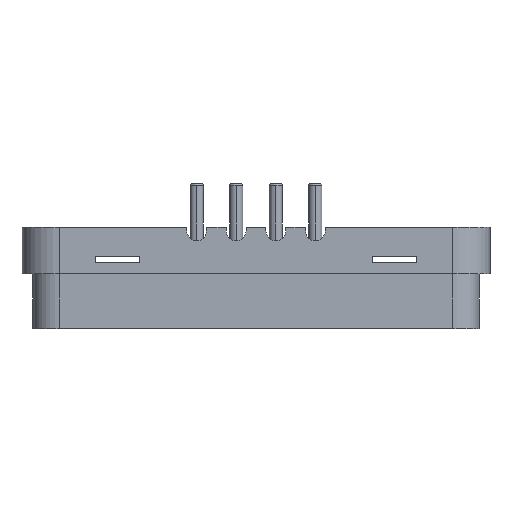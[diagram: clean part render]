
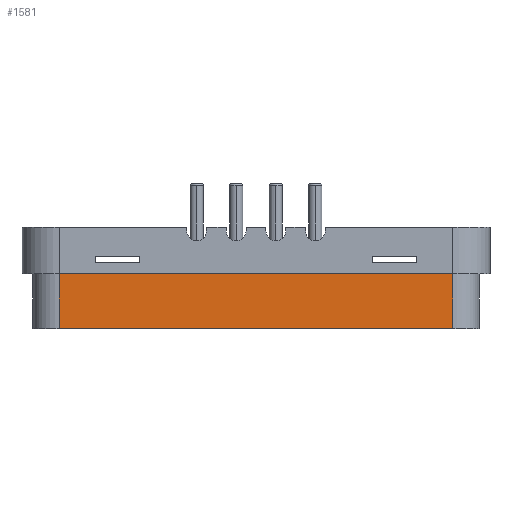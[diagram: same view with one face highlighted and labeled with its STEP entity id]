
A CAD part, front view. The second image highlights one B-rep face of the part: STEP entity #1581.
In plain terms, the highlighted planar face has unit normal (0, -1, 0).
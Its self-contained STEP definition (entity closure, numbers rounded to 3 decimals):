
#60 = LINE ( 'NONE', #7658, #10150 ) ;
#116 = CARTESIAN_POINT ( 'NONE',  ( -8.95, 18.25, 10.8 ) ) ;
#171 = ORIENTED_EDGE ( 'NONE', *, *, #3483, .F. ) ;
#277 = VERTEX_POINT ( 'NONE', #10784 ) ;
#297 = DIRECTION ( 'NONE',  ( 0., 0., 1. ) ) ;
#661 = DIRECTION ( 'NONE',  ( 0., 0., -1. ) ) ;
#1581 = ADVANCED_FACE ( 'NONE', ( #5797 ), #4277, .T. ) ;
#1880 = VERTEX_POINT ( 'NONE', #11144 ) ;
#2344 = CARTESIAN_POINT ( 'NONE',  ( -8.2, 18.25, 10.8 ) ) ;
#2667 = CARTESIAN_POINT ( 'NONE',  ( -8.95, 18.25, 13.3 ) ) ;
#3191 = AXIS2_PLACEMENT_3D ( 'NONE', #2344, #4167, #661 ) ;
#3281 = DIRECTION ( 'NONE',  ( 1., 0., 0. ) ) ;
#3436 = ORIENTED_EDGE ( 'NONE', *, *, #4422, .F. ) ;
#3483 = EDGE_CURVE ( 'NONE', #4690, #1880, #60, .T. ) ;
#3681 = CARTESIAN_POINT ( 'NONE',  ( 8.95, 18.25, 10.8 ) ) ;
#4003 = EDGE_LOOP ( 'NONE', ( #171, #10423, #3436, #6825 ) ) ;
#4167 = DIRECTION ( 'NONE',  ( 0., -1., 0. ) ) ;
#4277 = PLANE ( 'NONE',  #3191 ) ;
#4422 = EDGE_CURVE ( 'NONE', #277, #5569, #6389, .T. ) ;
#4587 = VECTOR ( 'NONE', #297, 1000. ) ;
#4690 = VERTEX_POINT ( 'NONE', #2667 ) ;
#5145 = EDGE_CURVE ( 'NONE', #277, #1880, #5448, .T. ) ;
#5448 = LINE ( 'NONE', #3681, #4587 ) ;
#5569 = VERTEX_POINT ( 'NONE', #116 ) ;
#5797 = FACE_OUTER_BOUND ( 'NONE', #4003, .T. ) ;
#5908 = LINE ( 'NONE', #9328, #9484 ) ;
#6389 = LINE ( 'NONE', #10447, #7381 ) ;
#6825 = ORIENTED_EDGE ( 'NONE', *, *, #5145, .T. ) ;
#7114 = DIRECTION ( 'NONE',  ( -1., 0., 0. ) ) ;
#7356 = DIRECTION ( 'NONE',  ( 0., 0., -1. ) ) ;
#7381 = VECTOR ( 'NONE', #7114, 1000. ) ;
#7388 = EDGE_CURVE ( 'NONE', #4690, #5569, #5908, .T. ) ;
#7658 = CARTESIAN_POINT ( 'NONE',  ( -8.95, 18.25, 13.3 ) ) ;
#9328 = CARTESIAN_POINT ( 'NONE',  ( -8.95, 18.25, 13.3 ) ) ;
#9484 = VECTOR ( 'NONE', #7356, 1000. ) ;
#10150 = VECTOR ( 'NONE', #3281, 1000. ) ;
#10423 = ORIENTED_EDGE ( 'NONE', *, *, #7388, .T. ) ;
#10447 = CARTESIAN_POINT ( 'NONE',  ( 8.95, 18.25, 10.8 ) ) ;
#10784 = CARTESIAN_POINT ( 'NONE',  ( 8.95, 18.25, 10.8 ) ) ;
#11144 = CARTESIAN_POINT ( 'NONE',  ( 8.95, 18.25, 13.3 ) ) ;
